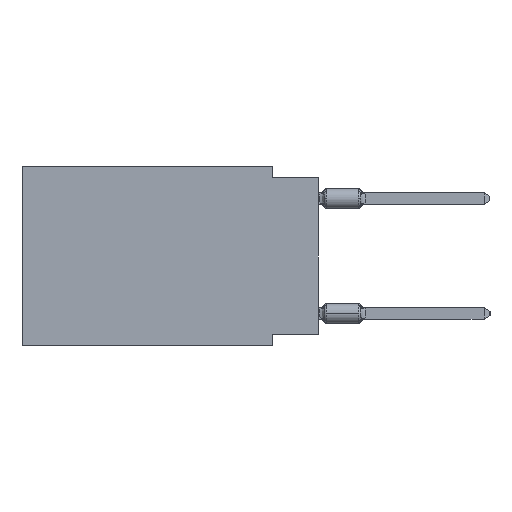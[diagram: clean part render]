
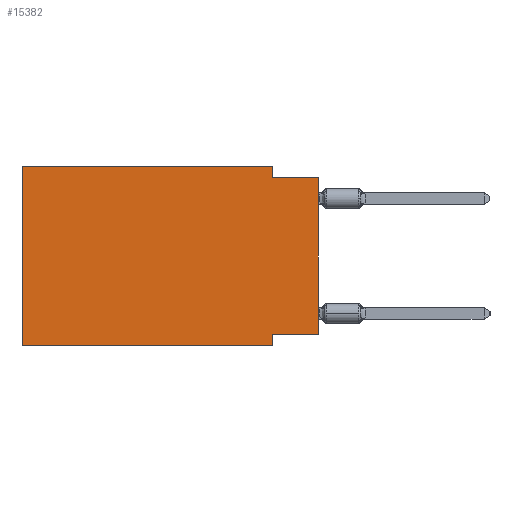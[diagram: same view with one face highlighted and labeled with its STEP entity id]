
A CAD part, left-side view. The second image highlights one B-rep face of the part: STEP entity #15382.
In plain terms, the highlighted planar face has unit normal (-1, 0, 0).
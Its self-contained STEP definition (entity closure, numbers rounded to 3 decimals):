
#654 = VERTEX_POINT ( 'NONE', #39305 ) ;
#1005 = ORIENTED_EDGE ( 'NONE', *, *, #30324, .F. ) ;
#2072 = CARTESIAN_POINT ( 'NONE',  ( 0., 16.383, 0. ) ) ;
#2273 = VERTEX_POINT ( 'NONE', #16662 ) ;
#2510 = DIRECTION ( 'NONE',  ( 0., 1., 0. ) ) ;
#2697 = VECTOR ( 'NONE', #32735, 1000. ) ;
#3369 = VECTOR ( 'NONE', #2510, 1000. ) ;
#3934 = DIRECTION ( 'NONE',  ( 0., -1., 0. ) ) ;
#4027 = LINE ( 'NONE', #38982, #41835 ) ;
#4526 = VERTEX_POINT ( 'NONE', #34570 ) ;
#4588 = DIRECTION ( 'NONE',  ( 0., 0., -1. ) ) ;
#4745 = ORIENTED_EDGE ( 'NONE', *, *, #29580, .F. ) ;
#5161 = DIRECTION ( 'NONE',  ( 0., -1., 0. ) ) ;
#6222 = CARTESIAN_POINT ( 'NONE',  ( 0., 16.383, 0. ) ) ;
#6999 = LINE ( 'NONE', #6222, #44934 ) ;
#7502 = VERTEX_POINT ( 'NONE', #45672 ) ;
#7957 = CARTESIAN_POINT ( 'NONE',  ( 0., 2.54, -9.271 ) ) ;
#8437 = DIRECTION ( 'NONE',  ( 1., 0., 0. ) ) ;
#8450 = CARTESIAN_POINT ( 'NONE',  ( 0., 0., -9.271 ) ) ;
#9195 = CARTESIAN_POINT ( 'NONE',  ( 0., 2.54, -9.906 ) ) ;
#11013 = VECTOR ( 'NONE', #48514, 1000. ) ;
#11534 = ORIENTED_EDGE ( 'NONE', *, *, #19869, .F. ) ;
#12505 = EDGE_CURVE ( 'NONE', #4526, #2273, #6999, .T. ) ;
#14218 = EDGE_LOOP ( 'NONE', ( #36214, #15509, #37528, #1005, #47470, #27538, #11534, #4745 ) ) ;
#14977 = DIRECTION ( 'NONE',  ( 0., 0., 1. ) ) ;
#15382 = ADVANCED_FACE ( 'NONE', ( #35919 ), #43652, .F. ) ;
#15509 = ORIENTED_EDGE ( 'NONE', *, *, #41273, .F. ) ;
#16662 = CARTESIAN_POINT ( 'NONE',  ( 0., 16.383, 0. ) ) ;
#17596 = VERTEX_POINT ( 'NONE', #37516 ) ;
#18936 = VECTOR ( 'NONE', #5161, 1000. ) ;
#19812 = CARTESIAN_POINT ( 'NONE',  ( 0., 16.383, -9.906 ) ) ;
#19869 = EDGE_CURVE ( 'NONE', #39270, #45878, #32803, .T. ) ;
#23461 = LINE ( 'NONE', #27316, #49175 ) ;
#24435 = CARTESIAN_POINT ( 'NONE',  ( 0., 2.54, -9.906 ) ) ;
#25059 = CARTESIAN_POINT ( 'NONE',  ( 0., 0., 0. ) ) ;
#27316 = CARTESIAN_POINT ( 'NONE',  ( 0., 0., -0.635 ) ) ;
#27538 = ORIENTED_EDGE ( 'NONE', *, *, #35333, .T. ) ;
#27953 = CARTESIAN_POINT ( 'NONE',  ( 0., 16.383, 0. ) ) ;
#29580 = EDGE_CURVE ( 'NONE', #43057, #39270, #40049, .T. ) ;
#29728 = EDGE_CURVE ( 'NONE', #654, #17596, #4027, .T. ) ;
#30324 = EDGE_CURVE ( 'NONE', #2273, #654, #36762, .T. ) ;
#30581 = LINE ( 'NONE', #19812, #42218 ) ;
#32425 = CARTESIAN_POINT ( 'NONE',  ( 0., 0., -9.271 ) ) ;
#32735 = DIRECTION ( 'NONE',  ( 0., 0., 1. ) ) ;
#32803 = LINE ( 'NONE', #9195, #11013 ) ;
#34570 = CARTESIAN_POINT ( 'NONE',  ( 0., 16.383, -9.906 ) ) ;
#35333 = EDGE_CURVE ( 'NONE', #4526, #45878, #30581, .T. ) ;
#35919 = FACE_OUTER_BOUND ( 'NONE', #14218, .T. ) ;
#36214 = ORIENTED_EDGE ( 'NONE', *, *, #49988, .T. ) ;
#36762 = LINE ( 'NONE', #2072, #18936 ) ;
#37516 = CARTESIAN_POINT ( 'NONE',  ( 0., 2.54, -0.635 ) ) ;
#37528 = ORIENTED_EDGE ( 'NONE', *, *, #29728, .F. ) ;
#38982 = CARTESIAN_POINT ( 'NONE',  ( 0., 2.54, 0. ) ) ;
#39270 = VERTEX_POINT ( 'NONE', #7957 ) ;
#39305 = CARTESIAN_POINT ( 'NONE',  ( 0., 2.54, 0. ) ) ;
#40049 = LINE ( 'NONE', #8450, #3369 ) ;
#41273 = EDGE_CURVE ( 'NONE', #17596, #7502, #23461, .T. ) ;
#41835 = VECTOR ( 'NONE', #50795, 1000. ) ;
#42218 = VECTOR ( 'NONE', #43190, 1000. ) ;
#43057 = VERTEX_POINT ( 'NONE', #32425 ) ;
#43190 = DIRECTION ( 'NONE',  ( 0., -1., 0. ) ) ;
#43652 = PLANE ( 'NONE',  #46956 ) ;
#44094 = LINE ( 'NONE', #25059, #2697 ) ;
#44934 = VECTOR ( 'NONE', #14977, 1000. ) ;
#45672 = CARTESIAN_POINT ( 'NONE',  ( 0., 0., -0.635 ) ) ;
#45878 = VERTEX_POINT ( 'NONE', #24435 ) ;
#46956 = AXIS2_PLACEMENT_3D ( 'NONE', #27953, #8437, #4588 ) ;
#47470 = ORIENTED_EDGE ( 'NONE', *, *, #12505, .F. ) ;
#48514 = DIRECTION ( 'NONE',  ( 0., 0., -1. ) ) ;
#49175 = VECTOR ( 'NONE', #3934, 1000. ) ;
#49988 = EDGE_CURVE ( 'NONE', #43057, #7502, #44094, .T. ) ;
#50795 = DIRECTION ( 'NONE',  ( 0., 0., -1. ) ) ;
